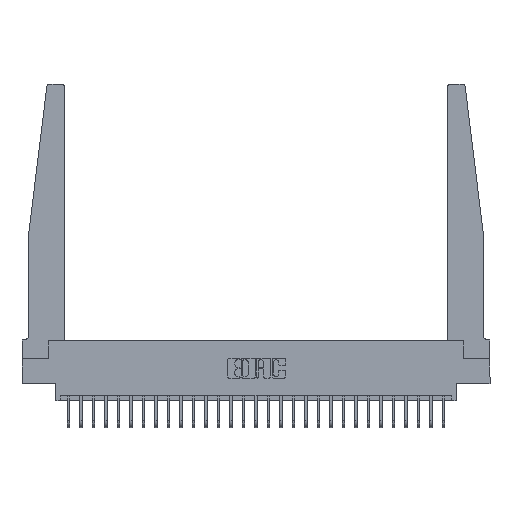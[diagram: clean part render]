
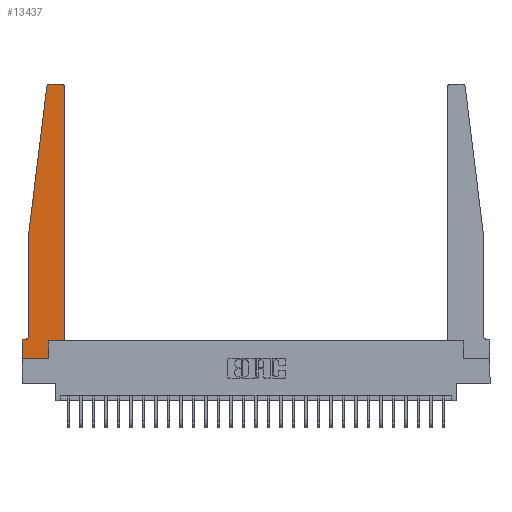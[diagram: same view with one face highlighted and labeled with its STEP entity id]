
A CAD part, top view. The second image highlights one B-rep face of the part: STEP entity #13437.
In plain terms, the highlighted planar face has unit normal (0, 0, 1).
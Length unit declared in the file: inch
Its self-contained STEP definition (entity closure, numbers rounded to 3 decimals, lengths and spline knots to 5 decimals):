
#226 = EDGE_CURVE ( 'NONE', #18461, #19909, #2676, .T. ) ;
#560 = VECTOR ( 'NONE', #13012, 39.37008 ) ;
#1258 = EDGE_CURVE ( 'NONE', #24551, #12597, #20019, .T. ) ;
#1672 = CARTESIAN_POINT ( 'NONE',  ( 0.065, 0.1875, 0.37 ) ) ;
#2676 = LINE ( 'NONE', #12885, #17333 ) ;
#3157 = EDGE_CURVE ( 'NONE', #16814, #18461, #5713, .T. ) ;
#3486 = DIRECTION ( 'NONE',  ( -1., 0., 0. ) ) ;
#3715 = CARTESIAN_POINT ( 'NONE',  ( 0., 0.1875, 0.37 ) ) ;
#3717 = DIRECTION ( 'NONE',  ( -1., 0., 0. ) ) ;
#3824 = LINE ( 'NONE', #14928, #19019 ) ;
#3836 = EDGE_CURVE ( 'NONE', #19909, #24551, #5986, .T. ) ;
#3986 = DIRECTION ( 'NONE',  ( 1., 0., 0. ) ) ;
#4333 = CARTESIAN_POINT ( 'NONE',  ( 0.2605, 0., 0.37 ) ) ;
#4570 = EDGE_CURVE ( 'NONE', #16702, #17372, #18705, .T. ) ;
#5713 = LINE ( 'NONE', #13837, #15656 ) ;
#5768 = ORIENTED_EDGE ( 'NONE', *, *, #3836, .T. ) ;
#5867 = CARTESIAN_POINT ( 'NONE',  ( 0.27653, 2.72, 0.37 ) ) ;
#5986 = LINE ( 'NONE', #22807, #560 ) ;
#6134 = CARTESIAN_POINT ( 'NONE',  ( 0.27653, 2.75, 0.37 ) ) ;
#6244 = ORIENTED_EDGE ( 'NONE', *, *, #4570, .T. ) ;
#6382 = ORIENTED_EDGE ( 'NONE', *, *, #10844, .T. ) ;
#6549 = EDGE_CURVE ( 'NONE', #7353, #16702, #7468, .T. ) ;
#6569 = CARTESIAN_POINT ( 'NONE',  ( 0.425, 0.18, 0.37 ) ) ;
#6649 = LINE ( 'NONE', #23181, #16588 ) ;
#6693 = CARTESIAN_POINT ( 'NONE',  ( 0.395, 2.75, 0.37 ) ) ;
#7353 = VERTEX_POINT ( 'NONE', #20427 ) ;
#7468 = CIRCLE ( 'NONE', #23438, 0.03 ) ;
#7471 = DIRECTION ( 'NONE',  ( -0.122, -0.992, 0. ) ) ;
#7703 = ORIENTED_EDGE ( 'NONE', *, *, #6549, .T. ) ;
#7871 = DIRECTION ( 'NONE',  ( 1., 0., 0. ) ) ;
#8062 = CARTESIAN_POINT ( 'NONE',  ( 0.395, 2.72, 0.37 ) ) ;
#8985 = CARTESIAN_POINT ( 'NONE',  ( 0.24675, 2.72367, 0.37 ) ) ;
#9071 = PLANE ( 'NONE',  #10492 ) ;
#9433 = CARTESIAN_POINT ( 'NONE',  ( 0.065, 1.25, 0.37 ) ) ;
#9451 = CARTESIAN_POINT ( 'NONE',  ( 0.25, 2.75, 0.37 ) ) ;
#10056 = DIRECTION ( 'NONE',  ( 1., 0., 0. ) ) ;
#10228 = CARTESIAN_POINT ( 'NONE',  ( 0.065, 1.25, 0.37 ) ) ;
#10492 = AXIS2_PLACEMENT_3D ( 'NONE', #20885, #22868, #11069 ) ;
#10832 = CIRCLE ( 'NONE', #15707, 0.03 ) ;
#10844 = EDGE_CURVE ( 'NONE', #12597, #7353, #3824, .T. ) ;
#10968 = VECTOR ( 'NONE', #14216, 39.37008 ) ;
#11008 = DIRECTION ( 'NONE',  ( 0., 1., 0. ) ) ;
#11069 = DIRECTION ( 'NONE',  ( 1., 0., 0. ) ) ;
#11089 = VECTOR ( 'NONE', #3717, 39.37008 ) ;
#11397 = CARTESIAN_POINT ( 'NONE',  ( 0.015, 0.1875, 0.37 ) ) ;
#11426 = FACE_OUTER_BOUND ( 'NONE', #18452, .T. ) ;
#11761 = ORIENTED_EDGE ( 'NONE', *, *, #226, .T. ) ;
#11915 = CARTESIAN_POINT ( 'NONE',  ( 0.015, 0.2375, 0.37 ) ) ;
#12093 = AXIS2_PLACEMENT_3D ( 'NONE', #11915, #25634, #13911 ) ;
#12597 = VERTEX_POINT ( 'NONE', #6569 ) ;
#12885 = CARTESIAN_POINT ( 'NONE',  ( 0., 0., 0.37 ) ) ;
#13012 = DIRECTION ( 'NONE',  ( 0., 1., 0. ) ) ;
#13435 = VERTEX_POINT ( 'NONE', #8985 ) ;
#13437 = ADVANCED_FACE ( 'NONE', ( #11426 ), #9071, .T. ) ;
#13604 = DIRECTION ( 'NONE',  ( 1., 0., 0. ) ) ;
#13675 = EDGE_CURVE ( 'NONE', #23308, #16814, #21572, .T. ) ;
#13837 = CARTESIAN_POINT ( 'NONE',  ( 0., 0., 0.37 ) ) ;
#13911 = DIRECTION ( 'NONE',  ( -1., 0., 0. ) ) ;
#14216 = DIRECTION ( 'NONE',  ( 0., -1., 0. ) ) ;
#14388 = VERTEX_POINT ( 'NONE', #20303 ) ;
#14462 = ORIENTED_EDGE ( 'NONE', *, *, #15967, .T. ) ;
#14928 = CARTESIAN_POINT ( 'NONE',  ( 0.425, 0.18, 0.37 ) ) ;
#15109 = ORIENTED_EDGE ( 'NONE', *, *, #3157, .T. ) ;
#15177 = ORIENTED_EDGE ( 'NONE', *, *, #13675, .T. ) ;
#15656 = VECTOR ( 'NONE', #23606, 39.37008 ) ;
#15707 = AXIS2_PLACEMENT_3D ( 'NONE', #5867, #19686, #7871 ) ;
#15967 = EDGE_CURVE ( 'NONE', #16342, #14388, #16842, .T. ) ;
#16342 = VERTEX_POINT ( 'NONE', #9433 ) ;
#16588 = VECTOR ( 'NONE', #7471, 39.37008 ) ;
#16702 = VERTEX_POINT ( 'NONE', #6693 ) ;
#16814 = VERTEX_POINT ( 'NONE', #3715 ) ;
#16842 = LINE ( 'NONE', #10228, #10968 ) ;
#17003 = ORIENTED_EDGE ( 'NONE', *, *, #1258, .T. ) ;
#17191 = CARTESIAN_POINT ( 'NONE',  ( 0.2605, 0.18, 0.37 ) ) ;
#17333 = VECTOR ( 'NONE', #13604, 39.37008 ) ;
#17372 = VERTEX_POINT ( 'NONE', #6134 ) ;
#18087 = VECTOR ( 'NONE', #3486, 39.37008 ) ;
#18452 = EDGE_LOOP ( 'NONE', ( #6244, #23667, #19741, #14462, #19675, #15177, #15109, #11761, #5768, #17003, #6382, #7703 ) ) ;
#18461 = VERTEX_POINT ( 'NONE', #23593 ) ;
#18705 = LINE ( 'NONE', #9451, #18087 ) ;
#19019 = VECTOR ( 'NONE', #11008, 39.37008 ) ;
#19675 = ORIENTED_EDGE ( 'NONE', *, *, #20622, .T. ) ;
#19686 = DIRECTION ( 'NONE',  ( 0., 0., 1. ) ) ;
#19741 = ORIENTED_EDGE ( 'NONE', *, *, #20592, .T. ) ;
#19909 = VERTEX_POINT ( 'NONE', #4333 ) ;
#20019 = LINE ( 'NONE', #25650, #25232 ) ;
#20303 = CARTESIAN_POINT ( 'NONE',  ( 0.065, 0.2375, 0.37 ) ) ;
#20427 = CARTESIAN_POINT ( 'NONE',  ( 0.425, 2.72, 0.37 ) ) ;
#20592 = EDGE_CURVE ( 'NONE', #13435, #16342, #6649, .T. ) ;
#20622 = EDGE_CURVE ( 'NONE', #14388, #23308, #21197, .T. ) ;
#20885 = CARTESIAN_POINT ( 'NONE',  ( 0., 0.1875, 0.37 ) ) ;
#21197 = CIRCLE ( 'NONE', #12093, 0.05 ) ;
#21572 = LINE ( 'NONE', #1672, #11089 ) ;
#21868 = DIRECTION ( 'NONE',  ( 0., 0., 1. ) ) ;
#22807 = CARTESIAN_POINT ( 'NONE',  ( 0.2605, 0.18, 0.37 ) ) ;
#22868 = DIRECTION ( 'NONE',  ( 0., 0., 1. ) ) ;
#23181 = CARTESIAN_POINT ( 'NONE',  ( 0.065, 1.25, 0.37 ) ) ;
#23308 = VERTEX_POINT ( 'NONE', #11397 ) ;
#23438 = AXIS2_PLACEMENT_3D ( 'NONE', #8062, #21868, #10056 ) ;
#23593 = CARTESIAN_POINT ( 'NONE',  ( 0., 0., 0.37 ) ) ;
#23606 = DIRECTION ( 'NONE',  ( 0., -1., 0. ) ) ;
#23667 = ORIENTED_EDGE ( 'NONE', *, *, #24091, .T. ) ;
#24091 = EDGE_CURVE ( 'NONE', #17372, #13435, #10832, .T. ) ;
#24551 = VERTEX_POINT ( 'NONE', #17191 ) ;
#25232 = VECTOR ( 'NONE', #3986, 39.37008 ) ;
#25634 = DIRECTION ( 'NONE',  ( 0., 0., -1. ) ) ;
#25650 = CARTESIAN_POINT ( 'NONE',  ( 0.425, 0.18, 0.37 ) ) ;
